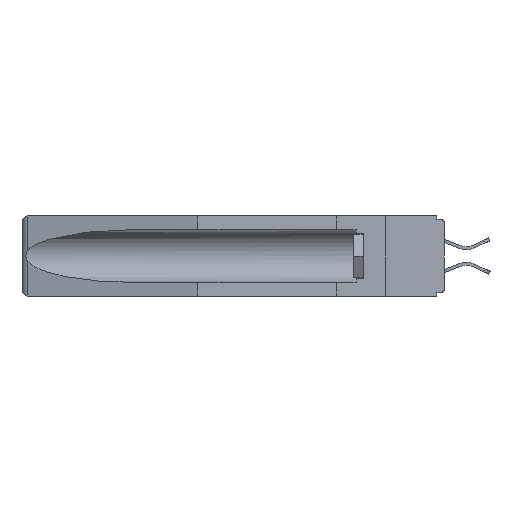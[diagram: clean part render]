
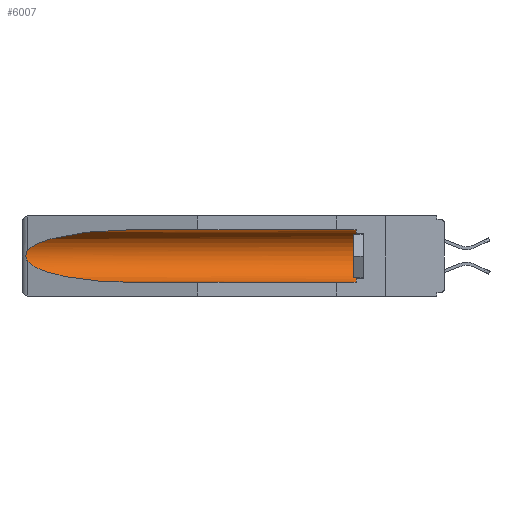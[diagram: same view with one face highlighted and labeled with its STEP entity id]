
A CAD part, left-side view. The second image highlights one B-rep face of the part: STEP entity #6007.
In plain terms, the highlighted cylindrical face has radius 2.857 mm (diameter 5.715 mm), a partial arc.
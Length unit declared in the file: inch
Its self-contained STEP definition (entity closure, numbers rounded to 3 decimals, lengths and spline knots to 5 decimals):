
#905 = CARTESIAN_POINT ( 'NONE',  ( 0.21114, 1.30732, -0.059 ) ) ;
#936 = CARTESIAN_POINT ( 'NONE',  ( 0.155, 1.07973, -0.284 ) ) ;
#1065 = AXIS2_PLACEMENT_3D ( 'NONE', #19159, #17932, #10223 ) ;
#1774 = ORIENTED_EDGE ( 'NONE', *, *, #8459, .T. ) ;
#1862 = CIRCLE ( 'NONE', #3730, 0.1125 ) ;
#2390 = CARTESIAN_POINT ( 'NONE',  ( 0.26537, 1.52718, -0.14972 ) ) ;
#2578 = CARTESIAN_POINT ( 'NONE',  ( 0.2675, 1.53308, -0.17534 ) ) ;
#2743 = VERTEX_POINT ( 'NONE', #4887 ) ;
#2842 = VERTEX_POINT ( 'NONE', #936 ) ;
#2863 = CARTESIAN_POINT ( 'NONE',  ( 0.155, -0.30754, -0.059 ) ) ;
#3127 = VERTEX_POINT ( 'NONE', #5968 ) ;
#3168 = B_SPLINE_CURVE_WITH_KNOTS ( 'NONE', 3,
 ( #3733, #17196, #8270, #12525, #18827, #2578, #17381, #14491, #14634, #8784 ),
 .UNSPECIFIED., .F., .F.,
 ( 4, 2, 2, 2, 4 ),
 ( 0., 0.00029, 0.00058, 0.00087, 0.00117 ),
 .UNSPECIFIED. ) ;
#3730 = AXIS2_PLACEMENT_3D ( 'NONE', #8600, #10340, #19009 ) ;
#3733 = CARTESIAN_POINT ( 'NONE',  ( 0.26537, 1.52718, -0.14972 ) ) ;
#4149 = EDGE_CURVE ( 'NONE', #3127, #14172, #3168, .T. ) ;
#4195 = LINE ( 'NONE', #2863, #8676 ) ;
#4475 = ORIENTED_EDGE ( 'NONE', *, *, #14982, .F. ) ;
#4543 = CARTESIAN_POINT ( 'NONE',  ( 0.25451, 1.48313, -0.24835 ) ) ;
#4657 = ORIENTED_EDGE ( 'NONE', *, *, #18958, .T. ) ;
#4887 = CARTESIAN_POINT ( 'NONE',  ( 0.155, 0.126, -0.059 ) ) ;
#5968 = CARTESIAN_POINT ( 'NONE',  ( 0.26537, 1.52718, -0.14972 ) ) ;
#6007 = ADVANCED_FACE ( 'NONE', ( #16313 ), #17717, .F. ) ;
#6254 = CARTESIAN_POINT ( 'NONE',  ( 0.21114, 1.30732, -0.284 ) ) ;
#6531 = ORIENTED_EDGE ( 'NONE', *, *, #13820, .T. ) ;
#7711 = VECTOR ( 'NONE', #19257, 39.37008 ) ;
#7888 =( BOUNDED_CURVE ( )  B_SPLINE_CURVE ( 3, ( #12153, #4543, #6254, #10505 ),
 .UNSPECIFIED., .F., .F. ) 
 B_SPLINE_CURVE_WITH_KNOTS ( ( 4, 4 ),
 ( 0.1948, 1.5708 ),
 .UNSPECIFIED. ) 
 CURVE ( )  GEOMETRIC_REPRESENTATION_ITEM ( )  RATIONAL_B_SPLINE_CURVE ( ( 1., 0.848, 0.848, 1. ) ) 
 REPRESENTATION_ITEM ( '' )  );
#8270 = CARTESIAN_POINT ( 'NONE',  ( 0.26654, 1.53092, -0.15636 ) ) ;
#8459 = EDGE_CURVE ( 'NONE', #11925, #3127, #18510, .T. ) ;
#8600 = CARTESIAN_POINT ( 'NONE',  ( 0.155, 0.126, -0.1715 ) ) ;
#8676 = VECTOR ( 'NONE', #10411, 39.37008 ) ;
#8784 = CARTESIAN_POINT ( 'NONE',  ( 0.26537, 1.52718, -0.19328 ) ) ;
#10189 = CARTESIAN_POINT ( 'NONE',  ( 0.155, -0.30754, -0.284 ) ) ;
#10223 = DIRECTION ( 'NONE',  ( 0., 0., 1. ) ) ;
#10340 = DIRECTION ( 'NONE',  ( 0., -1., 0. ) ) ;
#10411 = DIRECTION ( 'NONE',  ( 0., 1., 0. ) ) ;
#10505 = CARTESIAN_POINT ( 'NONE',  ( 0.155, 1.07973, -0.284 ) ) ;
#11387 = CARTESIAN_POINT ( 'NONE',  ( 0.25451, 1.48313, -0.09465 ) ) ;
#11925 = VERTEX_POINT ( 'NONE', #14114 ) ;
#12153 = CARTESIAN_POINT ( 'NONE',  ( 0.26537, 1.52718, -0.19328 ) ) ;
#12525 = CARTESIAN_POINT ( 'NONE',  ( 0.2673, 1.5327, -0.16383 ) ) ;
#13243 = EDGE_CURVE ( 'NONE', #14172, #2842, #7888, .T. ) ;
#13732 = ORIENTED_EDGE ( 'NONE', *, *, #4149, .T. ) ;
#13820 = EDGE_CURVE ( 'NONE', #2743, #11925, #4195, .T. ) ;
#14114 = CARTESIAN_POINT ( 'NONE',  ( 0.155, 1.07973, -0.059 ) ) ;
#14172 = VERTEX_POINT ( 'NONE', #18875 ) ;
#14491 = CARTESIAN_POINT ( 'NONE',  ( 0.26655, 1.53094, -0.18657 ) ) ;
#14634 = CARTESIAN_POINT ( 'NONE',  ( 0.26597, 1.5296, -0.19026 ) ) ;
#14917 = CARTESIAN_POINT ( 'NONE',  ( 0.155, 0.126, -0.284 ) ) ;
#14982 = EDGE_CURVE ( 'NONE', #18579, #2842, #18197, .T. ) ;
#15926 = EDGE_LOOP ( 'NONE', ( #1774, #13732, #17994, #4475, #4657, #6531 ) ) ;
#16313 = FACE_OUTER_BOUND ( 'NONE', #15926, .T. ) ;
#17196 = CARTESIAN_POINT ( 'NONE',  ( 0.26597, 1.52961, -0.15275 ) ) ;
#17381 = CARTESIAN_POINT ( 'NONE',  ( 0.2673, 1.53269, -0.17917 ) ) ;
#17717 = CYLINDRICAL_SURFACE ( 'NONE', #1065, 0.1125 ) ;
#17932 = DIRECTION ( 'NONE',  ( 0., 1., 0. ) ) ;
#17994 = ORIENTED_EDGE ( 'NONE', *, *, #13243, .T. ) ;
#18197 = LINE ( 'NONE', #10189, #7711 ) ;
#18510 =( BOUNDED_CURVE ( )  B_SPLINE_CURVE ( 3, ( #18828, #905, #11387, #2390 ),
 .UNSPECIFIED., .F., .F. ) 
 B_SPLINE_CURVE_WITH_KNOTS ( ( 4, 4 ),
 ( 4.71239, 6.08839 ),
 .UNSPECIFIED. ) 
 CURVE ( )  GEOMETRIC_REPRESENTATION_ITEM ( )  RATIONAL_B_SPLINE_CURVE ( ( 1., 0.848, 0.848, 1. ) ) 
 REPRESENTATION_ITEM ( '' )  );
#18579 = VERTEX_POINT ( 'NONE', #14917 ) ;
#18827 = CARTESIAN_POINT ( 'NONE',  ( 0.2675, 1.53308, -0.16763 ) ) ;
#18828 = CARTESIAN_POINT ( 'NONE',  ( 0.155, 1.07973, -0.059 ) ) ;
#18875 = CARTESIAN_POINT ( 'NONE',  ( 0.26537, 1.52718, -0.19328 ) ) ;
#18958 = EDGE_CURVE ( 'NONE', #18579, #2743, #1862, .T. ) ;
#19009 = DIRECTION ( 'NONE',  ( 0., 0., 1. ) ) ;
#19159 = CARTESIAN_POINT ( 'NONE',  ( 0.155, -0.30754, -0.1715 ) ) ;
#19257 = DIRECTION ( 'NONE',  ( 0., 1., 0. ) ) ;
